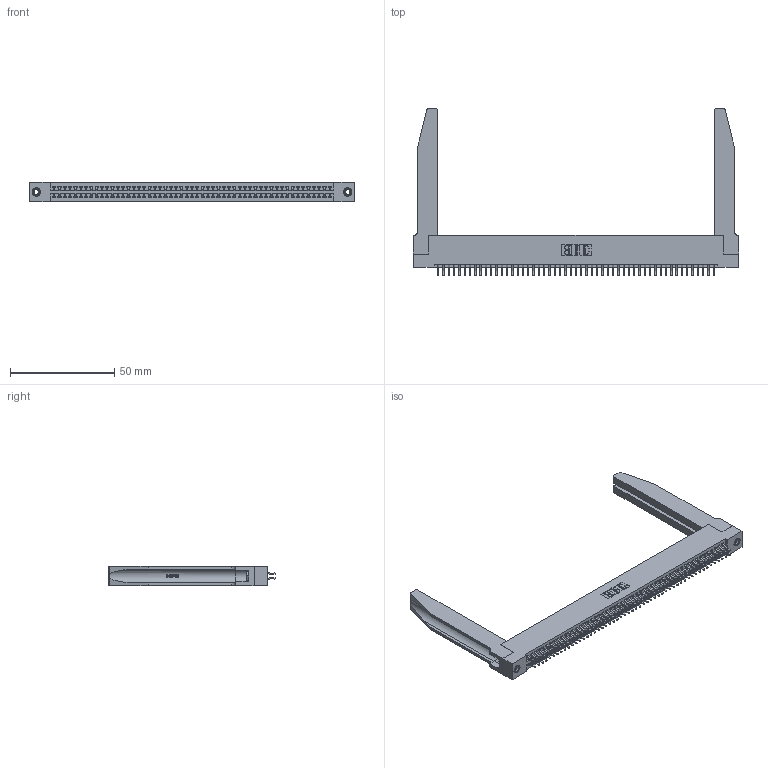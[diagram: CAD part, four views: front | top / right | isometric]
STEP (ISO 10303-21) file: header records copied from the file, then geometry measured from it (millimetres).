
FILE_DESCRIPTION (( 'STEP AP203' ), '1' );
FILE_NAME ('395-106-556-278.STEP', '2019-10-27T06:02:54', ( '' ), ( '' ), 'SwSTEP 2.0', 'SolidWorks 2016', '' );
FILE_SCHEMA (( 'CONFIG_CONTROL_DESIGN' ));
Length unit declared in the file: inch
Products named in the file (5): 345 Part_Flush Mounting Lugs - 0.156 Dia-TH; 345-292-001_556 Tail; 345-250-001_345-250-001-102; 345-220-078_345-220-078; 395-106-556-278
Assembly tree (111 placements, depth 2):
  395-106-556-278
    345 Part_Flush Mounting Lugs - 0.156 Dia-TH
    345-292-001_556 Tail  x106
    345-250-001_345-250-001-102  x2
    345-220-078_345-220-078  x2
Bounding box: 155.85 x 80.2 x 9.4 mm (x, y, z)
Volume: 23008.2 mm3; surface area: 29482.7 mm2
Topology: 111 solids, 111 shells, 6296 faces, 18651 edges, 12282 vertices
Faces by surface type: plane 4144, cylinder 2100, bspline 36, cone 12, torus 4
Entity records: 45064 total; most frequent: CARTESIAN_POINT 8475, ORIENTED_EDGE 7294, DIRECTION 6441, EDGE_CURVE 3647, VECTOR 3201, LINE 3201, VERTEX_POINT 2424, AXIS2_PLACEMENT_3D 1620
